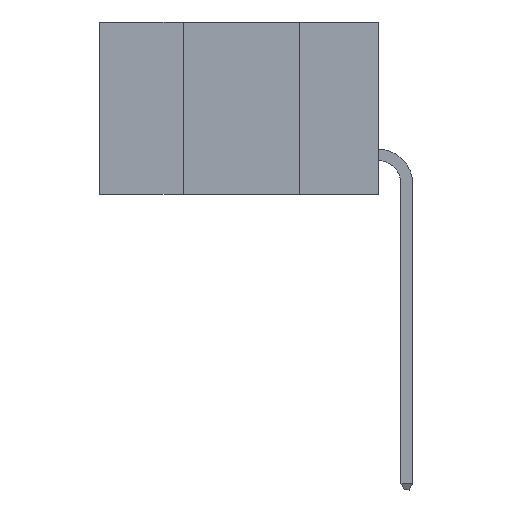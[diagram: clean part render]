
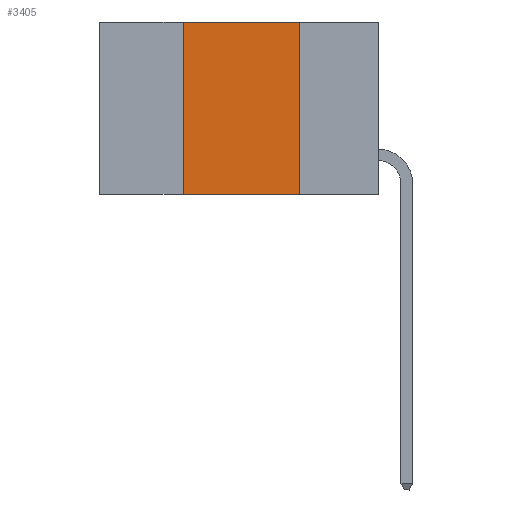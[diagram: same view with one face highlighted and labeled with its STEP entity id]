
A CAD part, left-side view. The second image highlights one B-rep face of the part: STEP entity #3405.
In plain terms, the highlighted planar face has unit normal (-1, 0, 0).
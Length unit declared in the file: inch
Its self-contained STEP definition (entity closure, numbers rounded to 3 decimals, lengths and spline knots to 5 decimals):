
#395 = FACE_OUTER_BOUND ( 'NONE', #15571, .T. ) ;
#799 = LINE ( 'NONE', #12712, #8266 ) ;
#844 = CARTESIAN_POINT ( 'NONE',  ( 0., 0.17, -0.37 ) ) ;
#1121 = AXIS2_PLACEMENT_3D ( 'NONE', #10989, #10279, #10218 ) ;
#1178 = EDGE_CURVE ( 'NONE', #7413, #2896, #17643, .T. ) ;
#1443 = VECTOR ( 'NONE', #18255, 39.37008 ) ;
#1771 = CARTESIAN_POINT ( 'NONE',  ( 0., 0.42, 0. ) ) ;
#2896 = VERTEX_POINT ( 'NONE', #844 ) ;
#2900 = CARTESIAN_POINT ( 'NONE',  ( 0., 0.17, 0. ) ) ;
#3405 = ADVANCED_FACE ( 'NONE', ( #395 ), #11254, .F. ) ;
#3798 = VERTEX_POINT ( 'NONE', #17413 ) ;
#4417 = DIRECTION ( 'NONE',  ( 0., 0., -1. ) ) ;
#5609 = ORIENTED_EDGE ( 'NONE', *, *, #1178, .T. ) ;
#5852 = EDGE_CURVE ( 'NONE', #13514, #3798, #799, .T. ) ;
#7293 = VECTOR ( 'NONE', #9276, 39.37008 ) ;
#7413 = VERTEX_POINT ( 'NONE', #14644 ) ;
#8266 = VECTOR ( 'NONE', #16841, 39.37008 ) ;
#8599 = ORIENTED_EDGE ( 'NONE', *, *, #5852, .F. ) ;
#9276 = DIRECTION ( 'NONE',  ( 0., 0., 1. ) ) ;
#9403 = VECTOR ( 'NONE', #4417, 39.37008 ) ;
#9570 = EDGE_CURVE ( 'NONE', #7413, #13514, #18973, .T. ) ;
#10218 = DIRECTION ( 'NONE',  ( 0., 0., -1. ) ) ;
#10279 = DIRECTION ( 'NONE',  ( 1., 0., 0. ) ) ;
#10989 = CARTESIAN_POINT ( 'NONE',  ( 0., 0.6, 0. ) ) ;
#11254 = PLANE ( 'NONE',  #1121 ) ;
#12077 = ORIENTED_EDGE ( 'NONE', *, *, #18968, .F. ) ;
#12712 = CARTESIAN_POINT ( 'NONE',  ( 0., 0.6, 0. ) ) ;
#13514 = VERTEX_POINT ( 'NONE', #15783 ) ;
#14644 = CARTESIAN_POINT ( 'NONE',  ( 0., 0.42, -0.37 ) ) ;
#15571 = EDGE_LOOP ( 'NONE', ( #12077, #8599, #16885, #5609 ) ) ;
#15783 = CARTESIAN_POINT ( 'NONE',  ( 0., 0.42, 0. ) ) ;
#16841 = DIRECTION ( 'NONE',  ( 0., -1., 0. ) ) ;
#16885 = ORIENTED_EDGE ( 'NONE', *, *, #9570, .F. ) ;
#17179 = LINE ( 'NONE', #2900, #9403 ) ;
#17413 = CARTESIAN_POINT ( 'NONE',  ( 0., 0.17, 0. ) ) ;
#17643 = LINE ( 'NONE', #18164, #1443 ) ;
#18164 = CARTESIAN_POINT ( 'NONE',  ( 0., 0.6, -0.37 ) ) ;
#18255 = DIRECTION ( 'NONE',  ( 0., -1., 0. ) ) ;
#18968 = EDGE_CURVE ( 'NONE', #3798, #2896, #17179, .T. ) ;
#18973 = LINE ( 'NONE', #1771, #7293 ) ;
